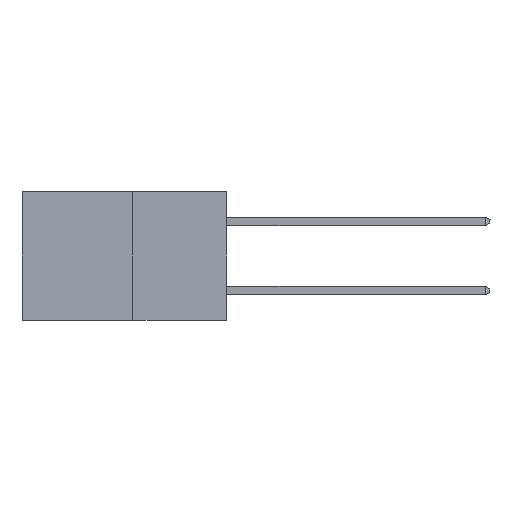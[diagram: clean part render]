
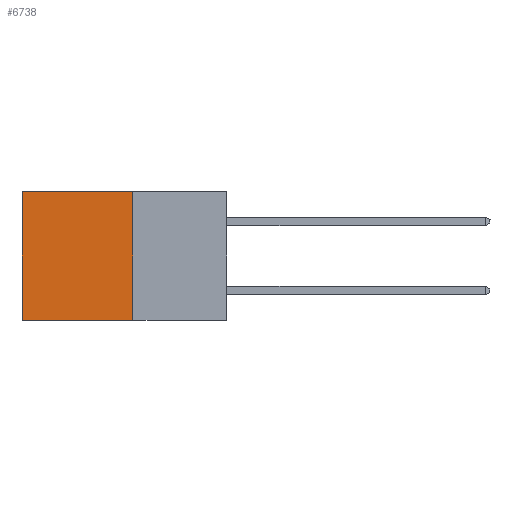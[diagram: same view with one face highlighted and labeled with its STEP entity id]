
A CAD part, left-side view. The second image highlights one B-rep face of the part: STEP entity #6738.
In plain terms, the highlighted planar face has unit normal (-1, 0, 0).
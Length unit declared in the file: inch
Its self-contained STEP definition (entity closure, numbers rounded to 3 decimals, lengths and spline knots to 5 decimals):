
#264 = CARTESIAN_POINT ( 'NONE',  ( 0.277, 0.27, 0. ) ) ;
#540 = VERTEX_POINT ( 'NONE', #10521 ) ;
#775 = LINE ( 'NONE', #859, #3162 ) ;
#823 = DIRECTION ( 'NONE',  ( 0., 1., 0. ) ) ;
#859 = CARTESIAN_POINT ( 'NONE',  ( 0.277, 0.27, -0.37 ) ) ;
#886 = EDGE_CURVE ( 'NONE', #5264, #2687, #7028, .T. ) ;
#1721 = EDGE_CURVE ( 'NONE', #540, #3816, #775, .T. ) ;
#1771 = LINE ( 'NONE', #4223, #10326 ) ;
#2201 = ORIENTED_EDGE ( 'NONE', *, *, #1721, .F. ) ;
#2687 = VERTEX_POINT ( 'NONE', #3572 ) ;
#3162 = VECTOR ( 'NONE', #6640, 39.37008 ) ;
#3224 = CARTESIAN_POINT ( 'NONE',  ( 0.277, 0.59, 0. ) ) ;
#3227 = ORIENTED_EDGE ( 'NONE', *, *, #886, .T. ) ;
#3572 = CARTESIAN_POINT ( 'NONE',  ( 0.277, 0.59, -0.37 ) ) ;
#3753 = ORIENTED_EDGE ( 'NONE', *, *, #8339, .F. ) ;
#3816 = VERTEX_POINT ( 'NONE', #7000 ) ;
#4223 = CARTESIAN_POINT ( 'NONE',  ( 0.277, 0.27, -0.37 ) ) ;
#4386 = VECTOR ( 'NONE', #11603, 39.37008 ) ;
#4580 = DIRECTION ( 'NONE',  ( 0., 0., -1. ) ) ;
#4681 = DIRECTION ( 'NONE',  ( 1., 0., 0. ) ) ;
#4745 = CARTESIAN_POINT ( 'NONE',  ( 0.277, 0.27, -0.37 ) ) ;
#4939 = CARTESIAN_POINT ( 'NONE',  ( 0.277, 0.59, -0.37 ) ) ;
#5081 = EDGE_LOOP ( 'NONE', ( #3227, #3753, #2201, #10897 ) ) ;
#5119 = FACE_OUTER_BOUND ( 'NONE', #5081, .T. ) ;
#5264 = VERTEX_POINT ( 'NONE', #3224 ) ;
#6598 = PLANE ( 'NONE',  #8854 ) ;
#6640 = DIRECTION ( 'NONE',  ( 0., 0., -1. ) ) ;
#6675 = VECTOR ( 'NONE', #11328, 39.37008 ) ;
#6738 = ADVANCED_FACE ( 'NONE', ( #5119 ), #6598, .F. ) ;
#7000 = CARTESIAN_POINT ( 'NONE',  ( 0.277, 0.27, -0.37 ) ) ;
#7028 = LINE ( 'NONE', #4939, #6675 ) ;
#7350 = LINE ( 'NONE', #264, #4386 ) ;
#8339 = EDGE_CURVE ( 'NONE', #3816, #2687, #1771, .T. ) ;
#8854 = AXIS2_PLACEMENT_3D ( 'NONE', #4745, #4681, #4580 ) ;
#10326 = VECTOR ( 'NONE', #823, 39.37008 ) ;
#10521 = CARTESIAN_POINT ( 'NONE',  ( 0.277, 0.27, 0. ) ) ;
#10897 = ORIENTED_EDGE ( 'NONE', *, *, #14241, .T. ) ;
#11328 = DIRECTION ( 'NONE',  ( 0., 0., -1. ) ) ;
#11603 = DIRECTION ( 'NONE',  ( 0., 1., 0. ) ) ;
#14241 = EDGE_CURVE ( 'NONE', #540, #5264, #7350, .T. ) ;
